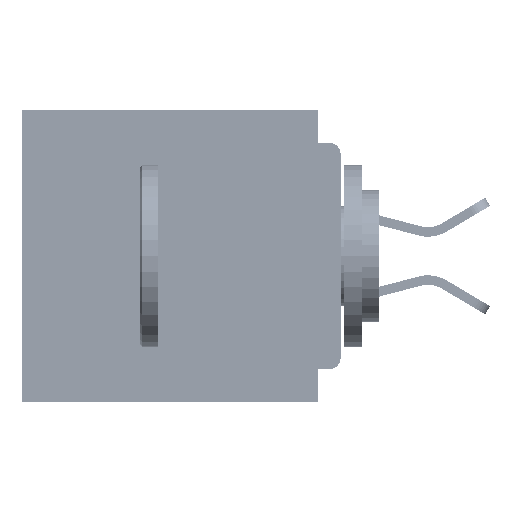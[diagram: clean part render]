
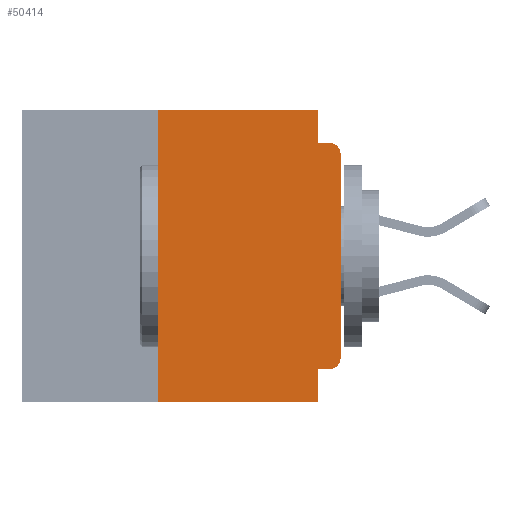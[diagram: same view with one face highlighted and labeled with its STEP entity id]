
A CAD part, left-side view. The second image highlights one B-rep face of the part: STEP entity #50414.
In plain terms, the highlighted planar face has unit normal (-1, 0, 0).
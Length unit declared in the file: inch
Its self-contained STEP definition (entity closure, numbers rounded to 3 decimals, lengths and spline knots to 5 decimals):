
#147 = VERTEX_POINT ( 'NONE', #28094 ) ;
#441 = VERTEX_POINT ( 'NONE', #56859 ) ;
#654 = AXIS2_PLACEMENT_3D ( 'NONE', #13114, #45440, #17765 ) ;
#845 = VECTOR ( 'NONE', #31405, 39.37008 ) ;
#1396 = CARTESIAN_POINT ( 'NONE',  ( 0., 0.437, 0. ) ) ;
#2659 = CARTESIAN_POINT ( 'NONE',  ( 0., 0.25, -0.4 ) ) ;
#3095 = ORIENTED_EDGE ( 'NONE', *, *, #52060, .F. ) ;
#4640 = CARTESIAN_POINT ( 'NONE',  ( 0., 0.031, 0. ) ) ;
#4673 = EDGE_LOOP ( 'NONE', ( #5548, #56709, #40667, #49629, #56834, #59619, #19246, #3095, #11140, #40489 ) ) ;
#4981 = VERTEX_POINT ( 'NONE', #52915 ) ;
#5158 = VERTEX_POINT ( 'NONE', #26421 ) ;
#5548 = ORIENTED_EDGE ( 'NONE', *, *, #14333, .T. ) ;
#5850 = DIRECTION ( 'NONE',  ( 0., 0., -1. ) ) ;
#6232 = DIRECTION ( 'NONE',  ( -1., 0., 0. ) ) ;
#6915 = CARTESIAN_POINT ( 'NONE',  ( 0., 0.437, -0.4 ) ) ;
#7270 = CARTESIAN_POINT ( 'NONE',  ( 0., 0.015, -0.355 ) ) ;
#7661 = CIRCLE ( 'NONE', #40097, 0.015 ) ;
#8390 = CARTESIAN_POINT ( 'NONE',  ( 0., 0., -0.355 ) ) ;
#9649 = DIRECTION ( 'NONE',  ( 0., -1., 0. ) ) ;
#10337 = CARTESIAN_POINT ( 'NONE',  ( 0., 0.031, 0. ) ) ;
#10445 = LINE ( 'NONE', #6915, #33598 ) ;
#11140 = ORIENTED_EDGE ( 'NONE', *, *, #41828, .F. ) ;
#11530 = VECTOR ( 'NONE', #42686, 39.37008 ) ;
#13114 = CARTESIAN_POINT ( 'NONE',  ( 0., 0.437, 0. ) ) ;
#14333 = EDGE_CURVE ( 'NONE', #147, #35600, #24331, .T. ) ;
#15155 = CARTESIAN_POINT ( 'NONE',  ( 0., 0.031, -0.4 ) ) ;
#16476 = EDGE_CURVE ( 'NONE', #39512, #147, #53619, .T. ) ;
#17524 = LINE ( 'NONE', #15155, #29807 ) ;
#17765 = DIRECTION ( 'NONE',  ( 0., 0., -1. ) ) ;
#18554 = VERTEX_POINT ( 'NONE', #44165 ) ;
#19246 = ORIENTED_EDGE ( 'NONE', *, *, #51548, .T. ) ;
#19665 = EDGE_CURVE ( 'NONE', #35600, #18554, #7661, .T. ) ;
#21416 = VERTEX_POINT ( 'NONE', #41393 ) ;
#22129 = FACE_OUTER_BOUND ( 'NONE', #4673, .T. ) ;
#24331 = LINE ( 'NONE', #37743, #35211 ) ;
#26421 = CARTESIAN_POINT ( 'NONE',  ( 0., 0.031, -0.045 ) ) ;
#26576 = DIRECTION ( 'NONE',  ( -1., 0., 0. ) ) ;
#26856 = LINE ( 'NONE', #8390, #845 ) ;
#28094 = CARTESIAN_POINT ( 'NONE',  ( 0., 0., -0.34 ) ) ;
#28516 = EDGE_CURVE ( 'NONE', #4981, #28828, #53871, .T. ) ;
#28828 = VERTEX_POINT ( 'NONE', #37237 ) ;
#29019 = EDGE_CURVE ( 'NONE', #28828, #59686, #50948, .T. ) ;
#29807 = VECTOR ( 'NONE', #5850, 39.37008 ) ;
#29883 = AXIS2_PLACEMENT_3D ( 'NONE', #54245, #26576, #58902 ) ;
#29962 = DIRECTION ( 'NONE',  ( 0., -1., 0. ) ) ;
#31090 = EDGE_CURVE ( 'NONE', #59686, #5158, #49851, .T. ) ;
#31405 = DIRECTION ( 'NONE',  ( 0., 1., 0. ) ) ;
#31758 = VECTOR ( 'NONE', #9649, 39.37008 ) ;
#33105 = DIRECTION ( 'NONE',  ( 0., 0., 1. ) ) ;
#33598 = VECTOR ( 'NONE', #29962, 39.37008 ) ;
#33840 = CARTESIAN_POINT ( 'NONE',  ( 0., 0., -0.06 ) ) ;
#33947 = CARTESIAN_POINT ( 'NONE',  ( 0., 0.015, -0.06 ) ) ;
#35011 = DIRECTION ( 'NONE',  ( 0., 0., 1. ) ) ;
#35211 = VECTOR ( 'NONE', #33105, 39.37008 ) ;
#35600 = VERTEX_POINT ( 'NONE', #33840 ) ;
#37237 = CARTESIAN_POINT ( 'NONE',  ( 0., 0.25, 0. ) ) ;
#37743 = CARTESIAN_POINT ( 'NONE',  ( 0., 0., 0. ) ) ;
#38409 = DIRECTION ( 'NONE',  ( 0., -1., 0. ) ) ;
#38600 = DIRECTION ( 'NONE',  ( 0., 0., -1. ) ) ;
#38670 = VECTOR ( 'NONE', #38409, 39.37008 ) ;
#39512 = VERTEX_POINT ( 'NONE', #7270 ) ;
#40097 = AXIS2_PLACEMENT_3D ( 'NONE', #33947, #6232, #38600 ) ;
#40489 = ORIENTED_EDGE ( 'NONE', *, *, #16476, .T. ) ;
#40667 = ORIENTED_EDGE ( 'NONE', *, *, #43207, .F. ) ;
#40831 = PLANE ( 'NONE',  #654 ) ;
#41393 = CARTESIAN_POINT ( 'NONE',  ( 0., 0.031, -0.4 ) ) ;
#41828 = EDGE_CURVE ( 'NONE', #39512, #441, #26856, .T. ) ;
#42686 = DIRECTION ( 'NONE',  ( 0., 0., -1. ) ) ;
#43207 = EDGE_CURVE ( 'NONE', #5158, #18554, #44078, .T. ) ;
#44078 = LINE ( 'NONE', #55710, #31758 ) ;
#44165 = CARTESIAN_POINT ( 'NONE',  ( 0., 0.015, -0.045 ) ) ;
#45440 = DIRECTION ( 'NONE',  ( 1., 0., 0. ) ) ;
#49629 = ORIENTED_EDGE ( 'NONE', *, *, #31090, .F. ) ;
#49851 = LINE ( 'NONE', #10337, #11530 ) ;
#50414 = ADVANCED_FACE ( 'NONE', ( #22129 ), #40831, .F. ) ;
#50948 = LINE ( 'NONE', #1396, #38670 ) ;
#51548 = EDGE_CURVE ( 'NONE', #4981, #21416, #10445, .T. ) ;
#52060 = EDGE_CURVE ( 'NONE', #441, #21416, #17524, .T. ) ;
#52915 = CARTESIAN_POINT ( 'NONE',  ( 0., 0.25, -0.4 ) ) ;
#53619 = CIRCLE ( 'NONE', #29883, 0.015 ) ;
#53871 = LINE ( 'NONE', #2659, #55328 ) ;
#54245 = CARTESIAN_POINT ( 'NONE',  ( 0., 0.015, -0.34 ) ) ;
#55328 = VECTOR ( 'NONE', #35011, 39.37008 ) ;
#55710 = CARTESIAN_POINT ( 'NONE',  ( 0., 0., -0.045 ) ) ;
#56709 = ORIENTED_EDGE ( 'NONE', *, *, #19665, .T. ) ;
#56834 = ORIENTED_EDGE ( 'NONE', *, *, #29019, .F. ) ;
#56859 = CARTESIAN_POINT ( 'NONE',  ( 0., 0.031, -0.355 ) ) ;
#58902 = DIRECTION ( 'NONE',  ( 0., 0., -1. ) ) ;
#59619 = ORIENTED_EDGE ( 'NONE', *, *, #28516, .F. ) ;
#59686 = VERTEX_POINT ( 'NONE', #4640 ) ;
